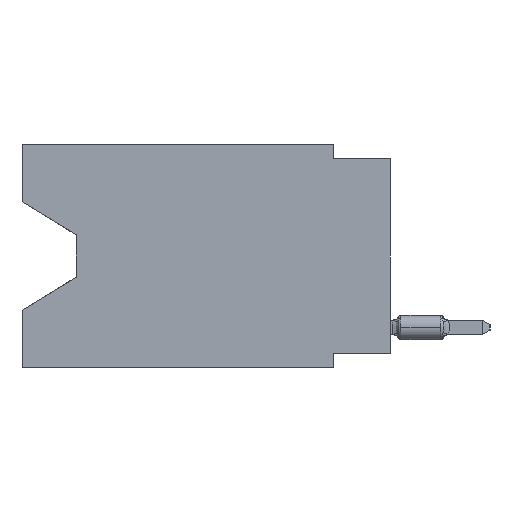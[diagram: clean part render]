
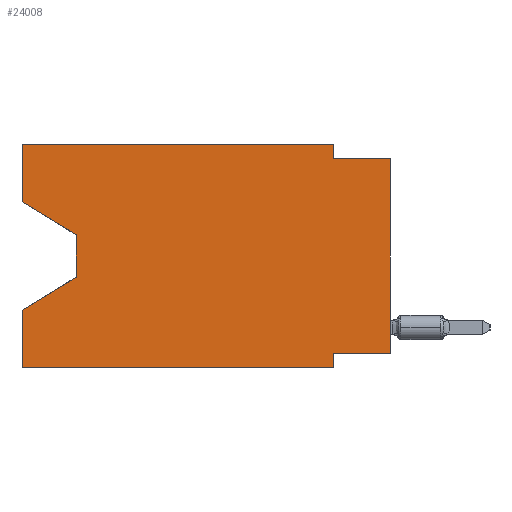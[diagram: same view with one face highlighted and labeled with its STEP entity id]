
A CAD part, left-side view. The second image highlights one B-rep face of the part: STEP entity #24008.
In plain terms, the highlighted planar face has unit normal (-1, 0, 0).
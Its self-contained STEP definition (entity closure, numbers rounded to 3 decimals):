
#109 = DIRECTION ( 'NONE',  ( 0., -1., 0. ) ) ;
#807 = CARTESIAN_POINT ( 'NONE',  ( 0., 13.97, -5.893 ) ) ;
#1405 = LINE ( 'NONE', #27592, #34839 ) ;
#1724 = VERTEX_POINT ( 'NONE', #36320 ) ;
#1980 = CARTESIAN_POINT ( 'NONE',  ( 0., 16.383, 0. ) ) ;
#2063 = CARTESIAN_POINT ( 'NONE',  ( 0., 0., 0. ) ) ;
#3016 = EDGE_CURVE ( 'NONE', #22126, #34965, #1405, .T. ) ;
#3544 = CARTESIAN_POINT ( 'NONE',  ( 0., 0., -9.271 ) ) ;
#4866 = VERTEX_POINT ( 'NONE', #37265 ) ;
#5141 = CARTESIAN_POINT ( 'NONE',  ( 0., 2.54, 0. ) ) ;
#5376 = FACE_OUTER_BOUND ( 'NONE', #22995, .T. ) ;
#5568 = CARTESIAN_POINT ( 'NONE',  ( 0., 16.383, 0. ) ) ;
#6042 = ORIENTED_EDGE ( 'NONE', *, *, #30098, .T. ) ;
#8315 = DIRECTION ( 'NONE',  ( 1., 0., 0. ) ) ;
#8770 = DIRECTION ( 'NONE',  ( 0., 0., -1. ) ) ;
#9207 = CARTESIAN_POINT ( 'NONE',  ( 0., 2.54, 0. ) ) ;
#9361 = DIRECTION ( 'NONE',  ( 0., -1., 0. ) ) ;
#9826 = CARTESIAN_POINT ( 'NONE',  ( 0., 13.97, -5.893 ) ) ;
#10323 = EDGE_CURVE ( 'NONE', #18358, #30437, #28430, .T. ) ;
#10723 = EDGE_CURVE ( 'NONE', #37488, #41012, #12467, .T. ) ;
#10963 = VECTOR ( 'NONE', #21082, 1000. ) ;
#11333 = VERTEX_POINT ( 'NONE', #37587 ) ;
#11972 = VECTOR ( 'NONE', #40077, 1000. ) ;
#12217 = PLANE ( 'NONE',  #36123 ) ;
#12467 = LINE ( 'NONE', #5141, #18836 ) ;
#12544 = ORIENTED_EDGE ( 'NONE', *, *, #30784, .T. ) ;
#13059 = EDGE_CURVE ( 'NONE', #31755, #31173, #20499, .T. ) ;
#13875 = VECTOR ( 'NONE', #109, 1000. ) ;
#14352 = CARTESIAN_POINT ( 'NONE',  ( 0., 16.383, 0. ) ) ;
#15739 = ORIENTED_EDGE ( 'NONE', *, *, #13059, .T. ) ;
#16008 = EDGE_CURVE ( 'NONE', #11333, #22126, #22144, .T. ) ;
#16883 = ORIENTED_EDGE ( 'NONE', *, *, #41373, .T. ) ;
#18233 = EDGE_CURVE ( 'NONE', #1724, #23474, #21720, .T. ) ;
#18358 = VERTEX_POINT ( 'NONE', #33468 ) ;
#18836 = VECTOR ( 'NONE', #20055, 1000. ) ;
#19116 = ORIENTED_EDGE ( 'NONE', *, *, #18233, .F. ) ;
#19554 = CARTESIAN_POINT ( 'NONE',  ( 0., 16.383, -7.36 ) ) ;
#20055 = DIRECTION ( 'NONE',  ( 0., 0., -1. ) ) ;
#20131 = LINE ( 'NONE', #27953, #46622 ) ;
#20499 = LINE ( 'NONE', #46715, #25918 ) ;
#21082 = DIRECTION ( 'NONE',  ( 0., 0., 1. ) ) ;
#21478 = ORIENTED_EDGE ( 'NONE', *, *, #10723, .F. ) ;
#21720 = LINE ( 'NONE', #1980, #37392 ) ;
#21903 = CARTESIAN_POINT ( 'NONE',  ( 0., 2.54, -9.906 ) ) ;
#22126 = VERTEX_POINT ( 'NONE', #25202 ) ;
#22144 = LINE ( 'NONE', #3544, #34533 ) ;
#22995 = EDGE_LOOP ( 'NONE', ( #6042, #15739, #43850, #19116, #16883, #34219, #47087, #12544, #38028, #21478, #37934, #31341 ) ) ;
#23079 = LINE ( 'NONE', #807, #35354 ) ;
#23241 = DIRECTION ( 'NONE',  ( 0., 0., -1. ) ) ;
#23474 = VERTEX_POINT ( 'NONE', #19554 ) ;
#23573 = CARTESIAN_POINT ( 'NONE',  ( 0., 0., -0.635 ) ) ;
#24008 = ADVANCED_FACE ( 'NONE', ( #5376 ), #12217, .F. ) ;
#24681 = EDGE_CURVE ( 'NONE', #31173, #23474, #23079, .T. ) ;
#25136 = LINE ( 'NONE', #5568, #11972 ) ;
#25202 = CARTESIAN_POINT ( 'NONE',  ( 0., 2.54, -9.271 ) ) ;
#25893 = EDGE_CURVE ( 'NONE', #30437, #37488, #25136, .T. ) ;
#25918 = VECTOR ( 'NONE', #8770, 1000. ) ;
#26521 = LINE ( 'NONE', #23573, #13875 ) ;
#27107 = VECTOR ( 'NONE', #28487, 1000. ) ;
#27592 = CARTESIAN_POINT ( 'NONE',  ( 0., 2.54, -9.906 ) ) ;
#27953 = CARTESIAN_POINT ( 'NONE',  ( 0., 16.383, -9.906 ) ) ;
#28430 = LINE ( 'NONE', #43372, #10963 ) ;
#28487 = DIRECTION ( 'NONE',  ( 0., 0., 1. ) ) ;
#29944 = DIRECTION ( 'NONE',  ( 0., 0.855, -0.519 ) ) ;
#30098 = EDGE_CURVE ( 'NONE', #18358, #31755, #43847, .T. ) ;
#30437 = VERTEX_POINT ( 'NONE', #14352 ) ;
#30784 = EDGE_CURVE ( 'NONE', #11333, #4866, #35586, .T. ) ;
#31173 = VERTEX_POINT ( 'NONE', #9826 ) ;
#31321 = CARTESIAN_POINT ( 'NONE',  ( 0., 16.383, 0. ) ) ;
#31341 = ORIENTED_EDGE ( 'NONE', *, *, #10323, .F. ) ;
#31755 = VERTEX_POINT ( 'NONE', #41290 ) ;
#32824 = CARTESIAN_POINT ( 'NONE',  ( 0., 16.383, -2.546 ) ) ;
#33468 = CARTESIAN_POINT ( 'NONE',  ( 0., 16.383, -2.546 ) ) ;
#34219 = ORIENTED_EDGE ( 'NONE', *, *, #3016, .F. ) ;
#34533 = VECTOR ( 'NONE', #47400, 1000. ) ;
#34839 = VECTOR ( 'NONE', #35908, 1000. ) ;
#34965 = VERTEX_POINT ( 'NONE', #21903 ) ;
#35354 = VECTOR ( 'NONE', #29944, 1000. ) ;
#35509 = DIRECTION ( 'NONE',  ( 0., 0., 1. ) ) ;
#35586 = LINE ( 'NONE', #2063, #27107 ) ;
#35908 = DIRECTION ( 'NONE',  ( 0., 0., -1. ) ) ;
#36123 = AXIS2_PLACEMENT_3D ( 'NONE', #31321, #8315, #23241 ) ;
#36320 = CARTESIAN_POINT ( 'NONE',  ( 0., 16.383, -9.906 ) ) ;
#37265 = CARTESIAN_POINT ( 'NONE',  ( 0., 0., -0.635 ) ) ;
#37392 = VECTOR ( 'NONE', #35509, 1000. ) ;
#37488 = VERTEX_POINT ( 'NONE', #9207 ) ;
#37587 = CARTESIAN_POINT ( 'NONE',  ( 0., 0., -9.271 ) ) ;
#37934 = ORIENTED_EDGE ( 'NONE', *, *, #25893, .F. ) ;
#38028 = ORIENTED_EDGE ( 'NONE', *, *, #42452, .F. ) ;
#38734 = VECTOR ( 'NONE', #43124, 1000. ) ;
#38789 = CARTESIAN_POINT ( 'NONE',  ( 0., 2.54, -0.635 ) ) ;
#40077 = DIRECTION ( 'NONE',  ( 0., -1., 0. ) ) ;
#41012 = VERTEX_POINT ( 'NONE', #38789 ) ;
#41290 = CARTESIAN_POINT ( 'NONE',  ( 0., 13.97, -4.013 ) ) ;
#41373 = EDGE_CURVE ( 'NONE', #1724, #34965, #20131, .T. ) ;
#42452 = EDGE_CURVE ( 'NONE', #41012, #4866, #26521, .T. ) ;
#43124 = DIRECTION ( 'NONE',  ( 0., -0.855, -0.519 ) ) ;
#43372 = CARTESIAN_POINT ( 'NONE',  ( 0., 16.383, 0. ) ) ;
#43847 = LINE ( 'NONE', #32824, #38734 ) ;
#43850 = ORIENTED_EDGE ( 'NONE', *, *, #24681, .T. ) ;
#46622 = VECTOR ( 'NONE', #9361, 1000. ) ;
#46715 = CARTESIAN_POINT ( 'NONE',  ( 0., 13.97, -4.013 ) ) ;
#47087 = ORIENTED_EDGE ( 'NONE', *, *, #16008, .F. ) ;
#47400 = DIRECTION ( 'NONE',  ( 0., 1., 0. ) ) ;
